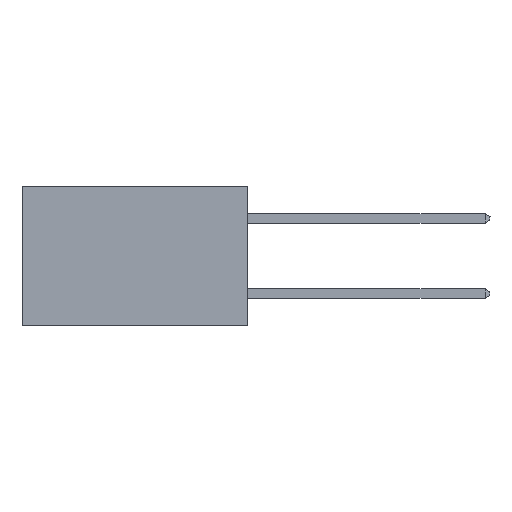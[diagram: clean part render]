
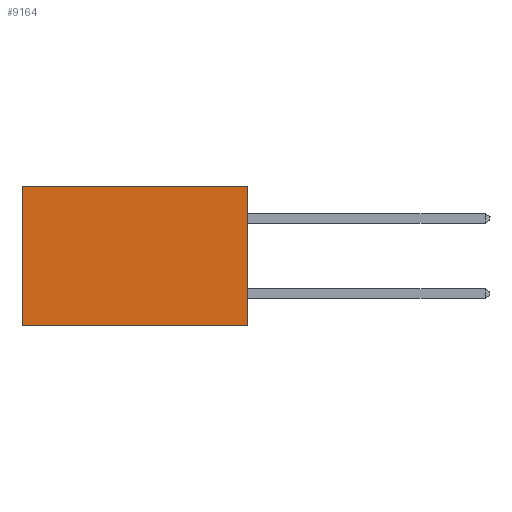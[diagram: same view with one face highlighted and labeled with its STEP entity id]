
A CAD part, left-side view. The second image highlights one B-rep face of the part: STEP entity #9164.
In plain terms, the highlighted planar face has unit normal (-1, 0, 0).
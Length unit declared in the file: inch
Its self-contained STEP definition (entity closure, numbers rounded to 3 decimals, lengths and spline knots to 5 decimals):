
#17 = VERTEX_POINT ( 'NONE', #311 ) ;
#311 = CARTESIAN_POINT ( 'NONE',  ( 0.298, 0., -0.37 ) ) ;
#703 = CARTESIAN_POINT ( 'NONE',  ( 0.298, 0., 0. ) ) ;
#1445 = PLANE ( 'NONE',  #5843 ) ;
#1473 = EDGE_CURVE ( 'NONE', #9115, #7486, #2864, .T. ) ;
#2050 = FACE_OUTER_BOUND ( 'NONE', #8241, .T. ) ;
#2127 = VECTOR ( 'NONE', #5455, 39.37008 ) ;
#2225 = ORIENTED_EDGE ( 'NONE', *, *, #3107, .T. ) ;
#2303 = EDGE_CURVE ( 'NONE', #17, #7486, #2494, .T. ) ;
#2314 = DIRECTION ( 'NONE',  ( 1., 0., 0. ) ) ;
#2343 = DIRECTION ( 'NONE',  ( 0., 0., -1. ) ) ;
#2494 = LINE ( 'NONE', #8401, #2127 ) ;
#2551 = DIRECTION ( 'NONE',  ( 0., 1., 0. ) ) ;
#2864 = LINE ( 'NONE', #4229, #7322 ) ;
#3107 = EDGE_CURVE ( 'NONE', #6074, #9115, #5500, .T. ) ;
#3435 = ORIENTED_EDGE ( 'NONE', *, *, #1473, .T. ) ;
#3600 = CARTESIAN_POINT ( 'NONE',  ( 0.298, 0.6, -0.37 ) ) ;
#3624 = CARTESIAN_POINT ( 'NONE',  ( 0.298, 0.6, 0. ) ) ;
#3702 = ORIENTED_EDGE ( 'NONE', *, *, #2303, .F. ) ;
#4229 = CARTESIAN_POINT ( 'NONE',  ( 0.298, 0.6, 0. ) ) ;
#4328 = ORIENTED_EDGE ( 'NONE', *, *, #6789, .F. ) ;
#5394 = VECTOR ( 'NONE', #2551, 39.37008 ) ;
#5455 = DIRECTION ( 'NONE',  ( 0., 1., 0. ) ) ;
#5500 = LINE ( 'NONE', #7021, #5394 ) ;
#5596 = CARTESIAN_POINT ( 'NONE',  ( 0.298, 0., 0. ) ) ;
#5843 = AXIS2_PLACEMENT_3D ( 'NONE', #703, #2314, #2343 ) ;
#6033 = CARTESIAN_POINT ( 'NONE',  ( 0.298, 0., 0. ) ) ;
#6074 = VERTEX_POINT ( 'NONE', #5596 ) ;
#6258 = LINE ( 'NONE', #6033, #7751 ) ;
#6789 = EDGE_CURVE ( 'NONE', #6074, #17, #6258, .T. ) ;
#7021 = CARTESIAN_POINT ( 'NONE',  ( 0.298, 0., 0. ) ) ;
#7322 = VECTOR ( 'NONE', #8723, 39.37008 ) ;
#7486 = VERTEX_POINT ( 'NONE', #3600 ) ;
#7751 = VECTOR ( 'NONE', #8886, 39.37008 ) ;
#8241 = EDGE_LOOP ( 'NONE', ( #3435, #3702, #4328, #2225 ) ) ;
#8401 = CARTESIAN_POINT ( 'NONE',  ( 0.298, 0., -0.37 ) ) ;
#8723 = DIRECTION ( 'NONE',  ( 0., 0., -1. ) ) ;
#8886 = DIRECTION ( 'NONE',  ( 0., 0., -1. ) ) ;
#9115 = VERTEX_POINT ( 'NONE', #3624 ) ;
#9164 = ADVANCED_FACE ( 'NONE', ( #2050 ), #1445, .F. ) ;
